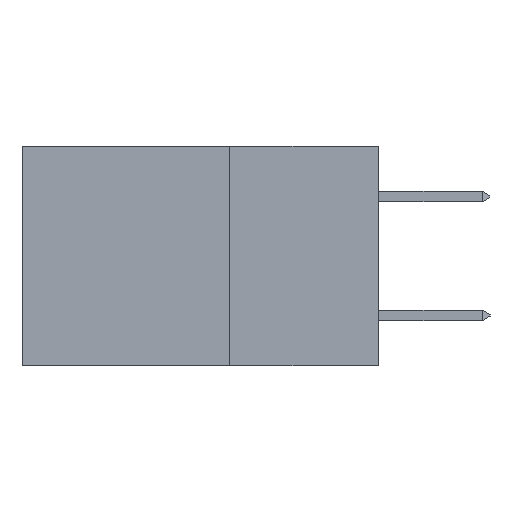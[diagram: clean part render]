
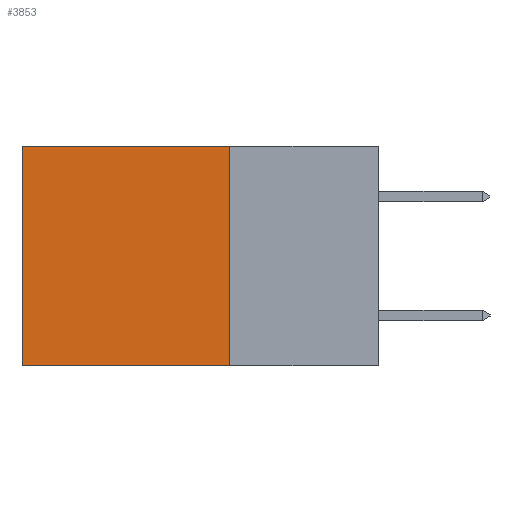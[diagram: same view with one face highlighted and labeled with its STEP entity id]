
A CAD part, left-side view. The second image highlights one B-rep face of the part: STEP entity #3853.
In plain terms, the highlighted planar face has unit normal (-1, 0, 0).
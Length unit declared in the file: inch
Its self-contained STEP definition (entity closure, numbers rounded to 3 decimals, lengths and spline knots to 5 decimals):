
#645 = DIRECTION ( 'NONE',  ( 0., 0., -1. ) ) ;
#705 = DIRECTION ( 'NONE',  ( 1., 0., 0. ) ) ;
#1191 = CARTESIAN_POINT ( 'NONE',  ( 0.2615, 0.25, -0.37 ) ) ;
#1338 = EDGE_CURVE ( 'NONE', #17648, #13107, #17769, .T. ) ;
#1342 = LINE ( 'NONE', #5501, #1881 ) ;
#1374 = PLANE ( 'NONE',  #20102 ) ;
#1622 = CARTESIAN_POINT ( 'NONE',  ( 0.2615, 0.25, -0.37 ) ) ;
#1881 = VECTOR ( 'NONE', #5232, 39.37008 ) ;
#3093 = LINE ( 'NONE', #9590, #6831 ) ;
#3782 = CARTESIAN_POINT ( 'NONE',  ( 0.2615, 0.25, 0. ) ) ;
#3852 = DIRECTION ( 'NONE',  ( 0., 1., 0. ) ) ;
#3853 = ADVANCED_FACE ( 'NONE', ( #5923 ), #1374, .F. ) ;
#4579 = CARTESIAN_POINT ( 'NONE',  ( 0.2615, 0.25, 0. ) ) ;
#4625 = EDGE_CURVE ( 'NONE', #10489, #4904, #1342, .T. ) ;
#4740 = EDGE_CURVE ( 'NONE', #10489, #17648, #7890, .T. ) ;
#4904 = VERTEX_POINT ( 'NONE', #1622 ) ;
#4917 = DIRECTION ( 'NONE',  ( 0., 1., 0. ) ) ;
#5232 = DIRECTION ( 'NONE',  ( 0., 0., -1. ) ) ;
#5501 = CARTESIAN_POINT ( 'NONE',  ( 0.2615, 0.25, -0.37 ) ) ;
#5923 = FACE_OUTER_BOUND ( 'NONE', #8028, .T. ) ;
#6533 = EDGE_CURVE ( 'NONE', #4904, #13107, #3093, .T. ) ;
#6831 = VECTOR ( 'NONE', #4917, 39.37008 ) ;
#7244 = ORIENTED_EDGE ( 'NONE', *, *, #4740, .T. ) ;
#7586 = ORIENTED_EDGE ( 'NONE', *, *, #6533, .F. ) ;
#7890 = LINE ( 'NONE', #3782, #15903 ) ;
#8028 = EDGE_LOOP ( 'NONE', ( #9711, #7586, #10459, #7244 ) ) ;
#9224 = VECTOR ( 'NONE', #19364, 39.37008 ) ;
#9590 = CARTESIAN_POINT ( 'NONE',  ( 0.2615, 0.25, -0.37 ) ) ;
#9711 = ORIENTED_EDGE ( 'NONE', *, *, #1338, .T. ) ;
#9712 = CARTESIAN_POINT ( 'NONE',  ( 0.2615, 0.6, -0.37 ) ) ;
#9976 = CARTESIAN_POINT ( 'NONE',  ( 0.2615, 0.6, 0. ) ) ;
#10459 = ORIENTED_EDGE ( 'NONE', *, *, #4625, .F. ) ;
#10489 = VERTEX_POINT ( 'NONE', #4579 ) ;
#13107 = VERTEX_POINT ( 'NONE', #9712 ) ;
#15903 = VECTOR ( 'NONE', #3852, 39.37008 ) ;
#17648 = VERTEX_POINT ( 'NONE', #9976 ) ;
#17769 = LINE ( 'NONE', #20080, #9224 ) ;
#19364 = DIRECTION ( 'NONE',  ( 0., 0., -1. ) ) ;
#20080 = CARTESIAN_POINT ( 'NONE',  ( 0.2615, 0.6, -0.37 ) ) ;
#20102 = AXIS2_PLACEMENT_3D ( 'NONE', #1191, #705, #645 ) ;
